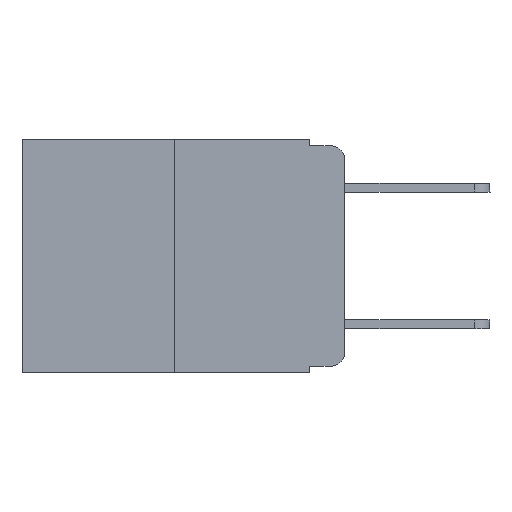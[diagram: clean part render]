
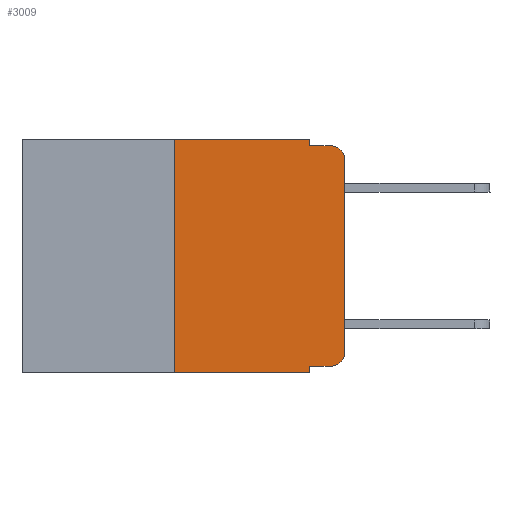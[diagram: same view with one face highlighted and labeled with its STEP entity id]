
A CAD part, left-side view. The second image highlights one B-rep face of the part: STEP entity #3009.
In plain terms, the highlighted planar face has unit normal (-1, 0, 0).
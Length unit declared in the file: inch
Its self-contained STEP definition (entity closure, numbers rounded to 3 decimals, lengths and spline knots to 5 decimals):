
#50 = CARTESIAN_POINT ( 'NONE',  ( 0., 0.473, 0. ) ) ;
#183 = VECTOR ( 'NONE', #16983, 39.37008 ) ;
#545 = CIRCLE ( 'NONE', #3822, 0.02 ) ;
#1012 = CARTESIAN_POINT ( 'NONE',  ( 0., 0.02, -0.333 ) ) ;
#1191 = ORIENTED_EDGE ( 'NONE', *, *, #3598, .F. ) ;
#1219 = CARTESIAN_POINT ( 'NONE',  ( 0., 0.02, -0.03 ) ) ;
#1374 = AXIS2_PLACEMENT_3D ( 'NONE', #50, #23287, #9960 ) ;
#1460 = CARTESIAN_POINT ( 'NONE',  ( 0., 0., -0.313 ) ) ;
#1643 = EDGE_LOOP ( 'NONE', ( #17052, #6703, #18960, #14312, #6971, #8192, #6862, #1191, #10190, #19077 ) ) ;
#1664 = CARTESIAN_POINT ( 'NONE',  ( 0., 0.25, 0. ) ) ;
#2113 = EDGE_CURVE ( 'NONE', #25081, #9785, #17138, .T. ) ;
#2176 = CARTESIAN_POINT ( 'NONE',  ( 0., 0.051, -0.01 ) ) ;
#2589 = CARTESIAN_POINT ( 'NONE',  ( 0., 0.051, 0. ) ) ;
#2812 = DIRECTION ( 'NONE',  ( 0., 0., -1. ) ) ;
#3009 = ADVANCED_FACE ( 'NONE', ( #17680 ), #19762, .F. ) ;
#3358 = VECTOR ( 'NONE', #7507, 39.37008 ) ;
#3598 = EDGE_CURVE ( 'NONE', #23254, #8881, #8390, .T. ) ;
#3822 = AXIS2_PLACEMENT_3D ( 'NONE', #1219, #22912, #11477 ) ;
#3853 = VECTOR ( 'NONE', #7634, 39.37008 ) ;
#5763 = CARTESIAN_POINT ( 'NONE',  ( 0., 0.02, -0.01 ) ) ;
#6703 = ORIENTED_EDGE ( 'NONE', *, *, #6978, .T. ) ;
#6862 = ORIENTED_EDGE ( 'NONE', *, *, #10461, .T. ) ;
#6888 = CARTESIAN_POINT ( 'NONE',  ( 0., 0.25, -0.343 ) ) ;
#6971 = ORIENTED_EDGE ( 'NONE', *, *, #12026, .F. ) ;
#6978 = EDGE_CURVE ( 'NONE', #9785, #24784, #545, .T. ) ;
#7507 = DIRECTION ( 'NONE',  ( 0., 0., -1. ) ) ;
#7518 = LINE ( 'NONE', #9557, #23019 ) ;
#7634 = DIRECTION ( 'NONE',  ( 0., 0., 1. ) ) ;
#7936 = CIRCLE ( 'NONE', #11209, 0.02 ) ;
#8192 = ORIENTED_EDGE ( 'NONE', *, *, #24271, .F. ) ;
#8347 = CARTESIAN_POINT ( 'NONE',  ( 0., 0.051, 0. ) ) ;
#8384 = VECTOR ( 'NONE', #14043, 39.37008 ) ;
#8390 = LINE ( 'NONE', #2589, #8384 ) ;
#8866 = DIRECTION ( 'NONE',  ( -1., 0., 0. ) ) ;
#8874 = VERTEX_POINT ( 'NONE', #2176 ) ;
#8881 = VERTEX_POINT ( 'NONE', #13635 ) ;
#9259 = LINE ( 'NONE', #25293, #183 ) ;
#9277 = VERTEX_POINT ( 'NONE', #1012 ) ;
#9557 = CARTESIAN_POINT ( 'NONE',  ( 0., 0.25, 0. ) ) ;
#9785 = VERTEX_POINT ( 'NONE', #21937 ) ;
#9868 = CARTESIAN_POINT ( 'NONE',  ( 0., 0.473, 0. ) ) ;
#9960 = DIRECTION ( 'NONE',  ( 0., 0., -1. ) ) ;
#10105 = VERTEX_POINT ( 'NONE', #1664 ) ;
#10190 = ORIENTED_EDGE ( 'NONE', *, *, #12588, .T. ) ;
#10461 = EDGE_CURVE ( 'NONE', #20071, #8881, #18901, .T. ) ;
#10726 = CARTESIAN_POINT ( 'NONE',  ( 0., 0.051, -0.01 ) ) ;
#11209 = AXIS2_PLACEMENT_3D ( 'NONE', #18651, #8866, #2812 ) ;
#11219 = CARTESIAN_POINT ( 'NONE',  ( 0., 0., 0. ) ) ;
#11477 = DIRECTION ( 'NONE',  ( 0., 0., -1. ) ) ;
#11812 = LINE ( 'NONE', #9868, #20310 ) ;
#12026 = EDGE_CURVE ( 'NONE', #10105, #12944, #11812, .T. ) ;
#12475 = VECTOR ( 'NONE', #20808, 39.37008 ) ;
#12588 = EDGE_CURVE ( 'NONE', #23254, #9277, #9259, .T. ) ;
#12922 = LINE ( 'NONE', #10726, #12475 ) ;
#12944 = VERTEX_POINT ( 'NONE', #8347 ) ;
#13635 = CARTESIAN_POINT ( 'NONE',  ( 0., 0.051, -0.343 ) ) ;
#13677 = CARTESIAN_POINT ( 'NONE',  ( 0., 0.051, 0. ) ) ;
#14043 = DIRECTION ( 'NONE',  ( 0., 0., -1. ) ) ;
#14312 = ORIENTED_EDGE ( 'NONE', *, *, #15428, .F. ) ;
#15420 = CARTESIAN_POINT ( 'NONE',  ( 0., 0.051, -0.333 ) ) ;
#15428 = EDGE_CURVE ( 'NONE', #12944, #8874, #19736, .T. ) ;
#16180 = EDGE_CURVE ( 'NONE', #9277, #25081, #7936, .T. ) ;
#16956 = CARTESIAN_POINT ( 'NONE',  ( 0., 0.473, -0.343 ) ) ;
#16983 = DIRECTION ( 'NONE',  ( 0., -1., 0. ) ) ;
#17052 = ORIENTED_EDGE ( 'NONE', *, *, #2113, .T. ) ;
#17138 = LINE ( 'NONE', #11219, #3853 ) ;
#17140 = EDGE_CURVE ( 'NONE', #8874, #24784, #12922, .T. ) ;
#17680 = FACE_OUTER_BOUND ( 'NONE', #1643, .T. ) ;
#17774 = VECTOR ( 'NONE', #22815, 39.37008 ) ;
#18651 = CARTESIAN_POINT ( 'NONE',  ( 0., 0.02, -0.313 ) ) ;
#18901 = LINE ( 'NONE', #16956, #17774 ) ;
#18960 = ORIENTED_EDGE ( 'NONE', *, *, #17140, .F. ) ;
#19077 = ORIENTED_EDGE ( 'NONE', *, *, #16180, .T. ) ;
#19736 = LINE ( 'NONE', #13677, #3358 ) ;
#19762 = PLANE ( 'NONE',  #1374 ) ;
#20071 = VERTEX_POINT ( 'NONE', #6888 ) ;
#20310 = VECTOR ( 'NONE', #23716, 39.37008 ) ;
#20808 = DIRECTION ( 'NONE',  ( 0., -1., 0. ) ) ;
#21692 = DIRECTION ( 'NONE',  ( 0., 0., 1. ) ) ;
#21937 = CARTESIAN_POINT ( 'NONE',  ( 0., 0., -0.03 ) ) ;
#22815 = DIRECTION ( 'NONE',  ( 0., -1., 0. ) ) ;
#22912 = DIRECTION ( 'NONE',  ( -1., 0., 0. ) ) ;
#23019 = VECTOR ( 'NONE', #21692, 39.37008 ) ;
#23254 = VERTEX_POINT ( 'NONE', #15420 ) ;
#23287 = DIRECTION ( 'NONE',  ( 1., 0., 0. ) ) ;
#23716 = DIRECTION ( 'NONE',  ( 0., -1., 0. ) ) ;
#24271 = EDGE_CURVE ( 'NONE', #20071, #10105, #7518, .T. ) ;
#24784 = VERTEX_POINT ( 'NONE', #5763 ) ;
#25081 = VERTEX_POINT ( 'NONE', #1460 ) ;
#25293 = CARTESIAN_POINT ( 'NONE',  ( 0., 0.051, -0.333 ) ) ;
